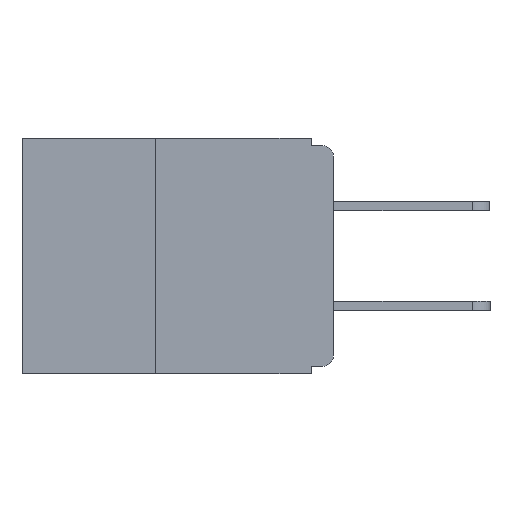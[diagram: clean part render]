
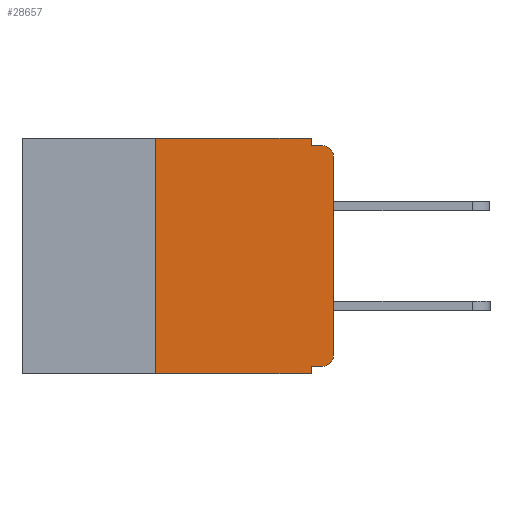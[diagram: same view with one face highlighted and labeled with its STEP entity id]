
A CAD part, left-side view. The second image highlights one B-rep face of the part: STEP entity #28657.
In plain terms, the highlighted planar face has unit normal (-1, 0, 0).
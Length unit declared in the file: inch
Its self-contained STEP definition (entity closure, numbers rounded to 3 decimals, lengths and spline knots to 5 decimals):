
#268 = LINE ( 'NONE', #23537, #16431 ) ;
#333 = CARTESIAN_POINT ( 'NONE',  ( 0., 0., -0.01 ) ) ;
#1012 = ORIENTED_EDGE ( 'NONE', *, *, #20501, .F. ) ;
#1198 = CARTESIAN_POINT ( 'NONE',  ( 0., 0.031, -0.01 ) ) ;
#1260 = DIRECTION ( 'NONE',  ( 0., 0., -1. ) ) ;
#1319 = EDGE_LOOP ( 'NONE', ( #10675, #17527, #26710, #1012, #4338, #10773, #12665, #12562, #14689, #6593 ) ) ;
#2175 = EDGE_CURVE ( 'NONE', #31449, #18564, #27486, .T. ) ;
#2291 = VECTOR ( 'NONE', #22991, 39.37008 ) ;
#3663 = AXIS2_PLACEMENT_3D ( 'NONE', #19041, #3697, #21505 ) ;
#3666 = LINE ( 'NONE', #333, #29651 ) ;
#3697 = DIRECTION ( 'NONE',  ( 1., 0., 0. ) ) ;
#4338 = ORIENTED_EDGE ( 'NONE', *, *, #8337, .F. ) ;
#4856 = CARTESIAN_POINT ( 'NONE',  ( 0., 0.031, 0. ) ) ;
#5201 = CARTESIAN_POINT ( 'NONE',  ( 0., 0.015, -0.025 ) ) ;
#5385 = CARTESIAN_POINT ( 'NONE',  ( 0., 0.015, -0.32 ) ) ;
#5505 = CARTESIAN_POINT ( 'NONE',  ( 0., 0.031, 0. ) ) ;
#5563 = DIRECTION ( 'NONE',  ( 0., -1., 0. ) ) ;
#5889 = CIRCLE ( 'NONE', #13799, 0.015 ) ;
#6014 = CARTESIAN_POINT ( 'NONE',  ( 0., 0., 0. ) ) ;
#6348 = EDGE_CURVE ( 'NONE', #31449, #20537, #268, .T. ) ;
#6593 = ORIENTED_EDGE ( 'NONE', *, *, #23947, .T. ) ;
#7468 = DIRECTION ( 'NONE',  ( 0., 0., -1. ) ) ;
#7822 = DIRECTION ( 'NONE',  ( 0., 0., -1. ) ) ;
#7945 = VECTOR ( 'NONE', #1260, 39.37008 ) ;
#8337 = EDGE_CURVE ( 'NONE', #18564, #21201, #22584, .T. ) ;
#8630 = DIRECTION ( 'NONE',  ( 0., 0., 1. ) ) ;
#9313 = VECTOR ( 'NONE', #14018, 39.37008 ) ;
#10097 = LINE ( 'NONE', #11399, #9313 ) ;
#10215 = VERTEX_POINT ( 'NONE', #28124 ) ;
#10675 = ORIENTED_EDGE ( 'NONE', *, *, #12328, .T. ) ;
#10773 = ORIENTED_EDGE ( 'NONE', *, *, #2175, .F. ) ;
#11399 = CARTESIAN_POINT ( 'NONE',  ( 0., 0., -0.32 ) ) ;
#12201 = LINE ( 'NONE', #4856, #24691 ) ;
#12328 = EDGE_CURVE ( 'NONE', #21754, #10215, #19608, .T. ) ;
#12562 = ORIENTED_EDGE ( 'NONE', *, *, #13983, .F. ) ;
#12665 = ORIENTED_EDGE ( 'NONE', *, *, #6348, .T. ) ;
#12917 = EDGE_CURVE ( 'NONE', #19396, #25927, #10097, .T. ) ;
#13799 = AXIS2_PLACEMENT_3D ( 'NONE', #5201, #22946, #7822 ) ;
#13935 = CARTESIAN_POINT ( 'NONE',  ( 0., 0.015, -0.305 ) ) ;
#13983 = EDGE_CURVE ( 'NONE', #25927, #20537, #21408, .T. ) ;
#14018 = DIRECTION ( 'NONE',  ( 0., 1., 0. ) ) ;
#14285 = EDGE_CURVE ( 'NONE', #10215, #30234, #5889, .T. ) ;
#14340 = VECTOR ( 'NONE', #31608, 39.37008 ) ;
#14689 = ORIENTED_EDGE ( 'NONE', *, *, #12917, .F. ) ;
#16431 = VECTOR ( 'NONE', #23768, 39.37008 ) ;
#16445 = DIRECTION ( 'NONE',  ( 0., 0., -1. ) ) ;
#17527 = ORIENTED_EDGE ( 'NONE', *, *, #14285, .T. ) ;
#18468 = CARTESIAN_POINT ( 'NONE',  ( 0., 0.031, -0.32 ) ) ;
#18564 = VERTEX_POINT ( 'NONE', #26181 ) ;
#19041 = CARTESIAN_POINT ( 'NONE',  ( 0., 0.437, 0. ) ) ;
#19396 = VERTEX_POINT ( 'NONE', #5385 ) ;
#19588 = VERTEX_POINT ( 'NONE', #1198 ) ;
#19608 = LINE ( 'NONE', #6014, #31817 ) ;
#20357 = CARTESIAN_POINT ( 'NONE',  ( 0., 0.031, -0.33 ) ) ;
#20501 = EDGE_CURVE ( 'NONE', #21201, #19588, #12201, .T. ) ;
#20505 = CARTESIAN_POINT ( 'NONE',  ( 0., 0.437, 0. ) ) ;
#20537 = VERTEX_POINT ( 'NONE', #20357 ) ;
#21201 = VERTEX_POINT ( 'NONE', #5505 ) ;
#21408 = LINE ( 'NONE', #31377, #7945 ) ;
#21505 = DIRECTION ( 'NONE',  ( 0., 0., -1. ) ) ;
#21754 = VERTEX_POINT ( 'NONE', #25463 ) ;
#22584 = LINE ( 'NONE', #20505, #2291 ) ;
#22938 = AXIS2_PLACEMENT_3D ( 'NONE', #13935, #31153, #16445 ) ;
#22946 = DIRECTION ( 'NONE',  ( -1., 0., 0. ) ) ;
#22991 = DIRECTION ( 'NONE',  ( 0., -1., 0. ) ) ;
#23537 = CARTESIAN_POINT ( 'NONE',  ( 0., 0.437, -0.33 ) ) ;
#23768 = DIRECTION ( 'NONE',  ( 0., -1., 0. ) ) ;
#23891 = PLANE ( 'NONE',  #3663 ) ;
#23947 = EDGE_CURVE ( 'NONE', #19396, #21754, #27183, .T. ) ;
#24691 = VECTOR ( 'NONE', #7468, 39.37008 ) ;
#25463 = CARTESIAN_POINT ( 'NONE',  ( 0., 0., -0.305 ) ) ;
#25927 = VERTEX_POINT ( 'NONE', #18468 ) ;
#26181 = CARTESIAN_POINT ( 'NONE',  ( 0., 0.25, 0. ) ) ;
#26710 = ORIENTED_EDGE ( 'NONE', *, *, #29622, .F. ) ;
#27183 = CIRCLE ( 'NONE', #22938, 0.015 ) ;
#27450 = CARTESIAN_POINT ( 'NONE',  ( 0., 0.25, -0.33 ) ) ;
#27486 = LINE ( 'NONE', #28224, #14340 ) ;
#27799 = FACE_OUTER_BOUND ( 'NONE', #1319, .T. ) ;
#27961 = CARTESIAN_POINT ( 'NONE',  ( 0., 0.015, -0.01 ) ) ;
#28124 = CARTESIAN_POINT ( 'NONE',  ( 0., 0., -0.025 ) ) ;
#28224 = CARTESIAN_POINT ( 'NONE',  ( 0., 0.25, -0.33 ) ) ;
#28657 = ADVANCED_FACE ( 'NONE', ( #27799 ), #23891, .F. ) ;
#29622 = EDGE_CURVE ( 'NONE', #19588, #30234, #3666, .T. ) ;
#29651 = VECTOR ( 'NONE', #5563, 39.37008 ) ;
#30234 = VERTEX_POINT ( 'NONE', #27961 ) ;
#31153 = DIRECTION ( 'NONE',  ( -1., 0., 0. ) ) ;
#31377 = CARTESIAN_POINT ( 'NONE',  ( 0., 0.031, -0.33 ) ) ;
#31449 = VERTEX_POINT ( 'NONE', #27450 ) ;
#31608 = DIRECTION ( 'NONE',  ( 0., 0., 1. ) ) ;
#31817 = VECTOR ( 'NONE', #8630, 39.37008 ) ;
